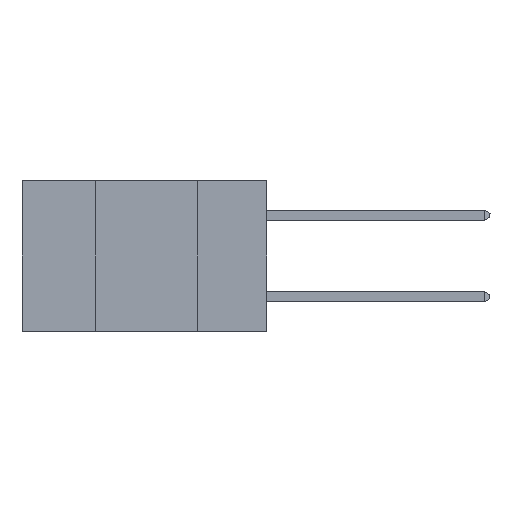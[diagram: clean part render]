
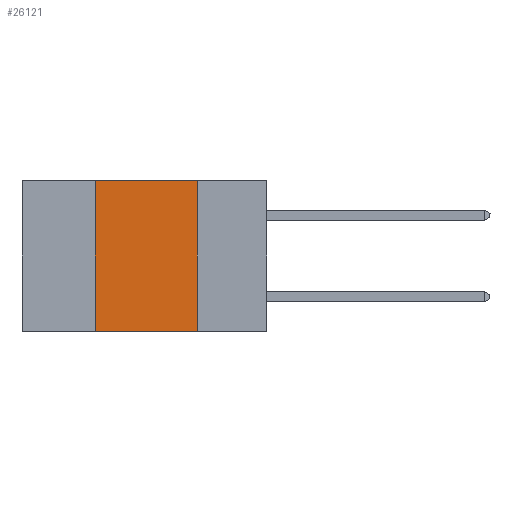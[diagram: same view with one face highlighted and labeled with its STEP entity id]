
A CAD part, left-side view. The second image highlights one B-rep face of the part: STEP entity #26121.
In plain terms, the highlighted planar face has unit normal (-1, 0, 0).
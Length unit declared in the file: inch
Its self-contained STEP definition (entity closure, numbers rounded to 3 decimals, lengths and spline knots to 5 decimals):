
#7 = CARTESIAN_POINT ( 'NONE',  ( 0., 0.6, 0. ) ) ;
#477 = VECTOR ( 'NONE', #26287, 39.37008 ) ;
#849 = LINE ( 'NONE', #26631, #8021 ) ;
#1632 = CARTESIAN_POINT ( 'NONE',  ( 0., 0.6, 0. ) ) ;
#1922 = CARTESIAN_POINT ( 'NONE',  ( 0., 0.17, -0.37 ) ) ;
#3998 = DIRECTION ( 'NONE',  ( 0., 0., -1. ) ) ;
#5609 = DIRECTION ( 'NONE',  ( 0., -1., 0. ) ) ;
#7121 = CARTESIAN_POINT ( 'NONE',  ( 0., 0.42, 0. ) ) ;
#7532 = LINE ( 'NONE', #7, #8507 ) ;
#7552 = EDGE_LOOP ( 'NONE', ( #9796, #15816, #8247, #16753 ) ) ;
#8021 = VECTOR ( 'NONE', #5609, 39.37008 ) ;
#8247 = ORIENTED_EDGE ( 'NONE', *, *, #12346, .F. ) ;
#8507 = VECTOR ( 'NONE', #9378, 39.37008 ) ;
#9146 = DIRECTION ( 'NONE',  ( 0., 0., -1. ) ) ;
#9281 = LINE ( 'NONE', #19255, #477 ) ;
#9378 = DIRECTION ( 'NONE',  ( 0., -1., 0. ) ) ;
#9796 = ORIENTED_EDGE ( 'NONE', *, *, #22507, .F. ) ;
#10796 = VECTOR ( 'NONE', #3998, 39.37008 ) ;
#10956 = VERTEX_POINT ( 'NONE', #7121 ) ;
#12078 = EDGE_CURVE ( 'NONE', #16262, #26114, #849, .T. ) ;
#12346 = EDGE_CURVE ( 'NONE', #16262, #10956, #9281, .T. ) ;
#13734 = CARTESIAN_POINT ( 'NONE',  ( 0., 0.17, 0. ) ) ;
#15237 = CARTESIAN_POINT ( 'NONE',  ( 0., 0.42, -0.37 ) ) ;
#15816 = ORIENTED_EDGE ( 'NONE', *, *, #28521, .F. ) ;
#16004 = CARTESIAN_POINT ( 'NONE',  ( 0., 0.17, 0. ) ) ;
#16262 = VERTEX_POINT ( 'NONE', #15237 ) ;
#16392 = PLANE ( 'NONE',  #21132 ) ;
#16753 = ORIENTED_EDGE ( 'NONE', *, *, #12078, .T. ) ;
#18216 = DIRECTION ( 'NONE',  ( 1., 0., 0. ) ) ;
#19255 = CARTESIAN_POINT ( 'NONE',  ( 0., 0.42, 0. ) ) ;
#20501 = FACE_OUTER_BOUND ( 'NONE', #7552, .T. ) ;
#21132 = AXIS2_PLACEMENT_3D ( 'NONE', #1632, #18216, #9146 ) ;
#22507 = EDGE_CURVE ( 'NONE', #26678, #26114, #27624, .T. ) ;
#26114 = VERTEX_POINT ( 'NONE', #1922 ) ;
#26121 = ADVANCED_FACE ( 'NONE', ( #20501 ), #16392, .F. ) ;
#26287 = DIRECTION ( 'NONE',  ( 0., 0., 1. ) ) ;
#26631 = CARTESIAN_POINT ( 'NONE',  ( 0., 0.6, -0.37 ) ) ;
#26678 = VERTEX_POINT ( 'NONE', #13734 ) ;
#27624 = LINE ( 'NONE', #16004, #10796 ) ;
#28521 = EDGE_CURVE ( 'NONE', #10956, #26678, #7532, .T. ) ;
